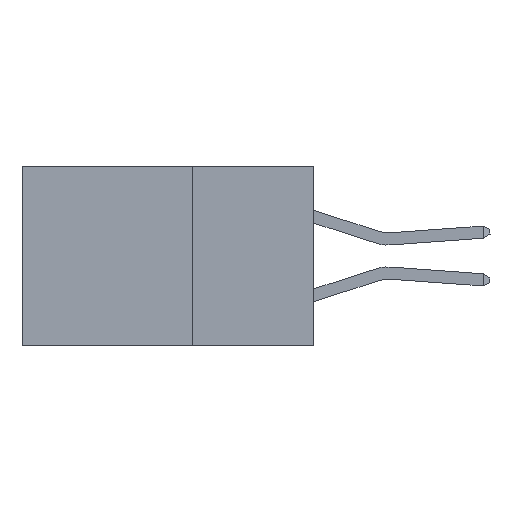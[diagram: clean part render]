
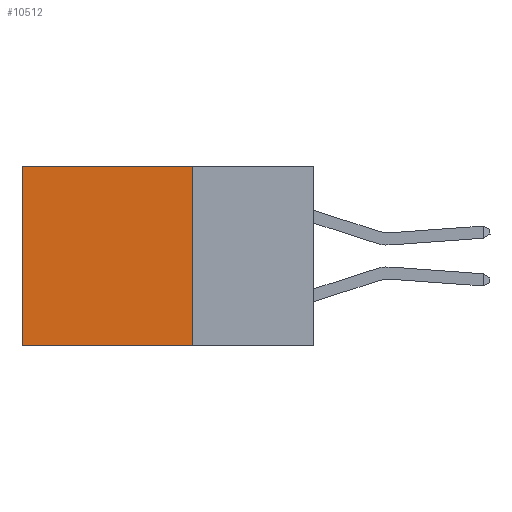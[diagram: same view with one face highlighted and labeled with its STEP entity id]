
A CAD part, left-side view. The second image highlights one B-rep face of the part: STEP entity #10512.
In plain terms, the highlighted planar face has unit normal (-1, 0, 0).
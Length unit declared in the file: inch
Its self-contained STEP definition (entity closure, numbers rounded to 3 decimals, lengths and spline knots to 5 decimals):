
#648 = ORIENTED_EDGE ( 'NONE', *, *, #12069, .T. ) ;
#825 = CARTESIAN_POINT ( 'NONE',  ( 0.2875, 0.25, 0. ) ) ;
#909 = VERTEX_POINT ( 'NONE', #2403 ) ;
#999 = VECTOR ( 'NONE', #7450, 39.37008 ) ;
#1350 = CARTESIAN_POINT ( 'NONE',  ( 0.2875, 0.6, 0. ) ) ;
#1523 = CARTESIAN_POINT ( 'NONE',  ( 0.2875, 0.25, 0. ) ) ;
#2271 = CARTESIAN_POINT ( 'NONE',  ( 0.2875, 0.6, 0. ) ) ;
#2403 = CARTESIAN_POINT ( 'NONE',  ( 0.2875, 0.6, -0.37 ) ) ;
#2502 = EDGE_CURVE ( 'NONE', #2829, #909, #8251, .T. ) ;
#2829 = VERTEX_POINT ( 'NONE', #9097 ) ;
#3225 = AXIS2_PLACEMENT_3D ( 'NONE', #825, #11714, #8241 ) ;
#3292 = EDGE_CURVE ( 'NONE', #9660, #2829, #8073, .T. ) ;
#3302 = LINE ( 'NONE', #11925, #999 ) ;
#3340 = LINE ( 'NONE', #2271, #11532 ) ;
#3649 = EDGE_CURVE ( 'NONE', #5625, #909, #3340, .T. ) ;
#3953 = VECTOR ( 'NONE', #10408, 39.37008 ) ;
#5625 = VERTEX_POINT ( 'NONE', #1350 ) ;
#6123 = CARTESIAN_POINT ( 'NONE',  ( 0.2875, 0.25, -0.37 ) ) ;
#6395 = ORIENTED_EDGE ( 'NONE', *, *, #3649, .T. ) ;
#6575 = DIRECTION ( 'NONE',  ( 0., 0., -1. ) ) ;
#7181 = ORIENTED_EDGE ( 'NONE', *, *, #2502, .F. ) ;
#7450 = DIRECTION ( 'NONE',  ( 0., 1., 0. ) ) ;
#7653 = VECTOR ( 'NONE', #11662, 39.37008 ) ;
#8073 = LINE ( 'NONE', #1523, #3953 ) ;
#8241 = DIRECTION ( 'NONE',  ( 0., 0., -1. ) ) ;
#8251 = LINE ( 'NONE', #6123, #7653 ) ;
#8271 = CARTESIAN_POINT ( 'NONE',  ( 0.2875, 0.25, 0. ) ) ;
#9097 = CARTESIAN_POINT ( 'NONE',  ( 0.2875, 0.25, -0.37 ) ) ;
#9593 = ORIENTED_EDGE ( 'NONE', *, *, #3292, .F. ) ;
#9660 = VERTEX_POINT ( 'NONE', #8271 ) ;
#9919 = EDGE_LOOP ( 'NONE', ( #6395, #7181, #9593, #648 ) ) ;
#10408 = DIRECTION ( 'NONE',  ( 0., 0., -1. ) ) ;
#10512 = ADVANCED_FACE ( 'NONE', ( #12637 ), #13833, .F. ) ;
#11532 = VECTOR ( 'NONE', #6575, 39.37008 ) ;
#11662 = DIRECTION ( 'NONE',  ( 0., 1., 0. ) ) ;
#11714 = DIRECTION ( 'NONE',  ( 1., 0., 0. ) ) ;
#11925 = CARTESIAN_POINT ( 'NONE',  ( 0.2875, 0.25, 0. ) ) ;
#12069 = EDGE_CURVE ( 'NONE', #9660, #5625, #3302, .T. ) ;
#12637 = FACE_OUTER_BOUND ( 'NONE', #9919, .T. ) ;
#13833 = PLANE ( 'NONE',  #3225 ) ;
